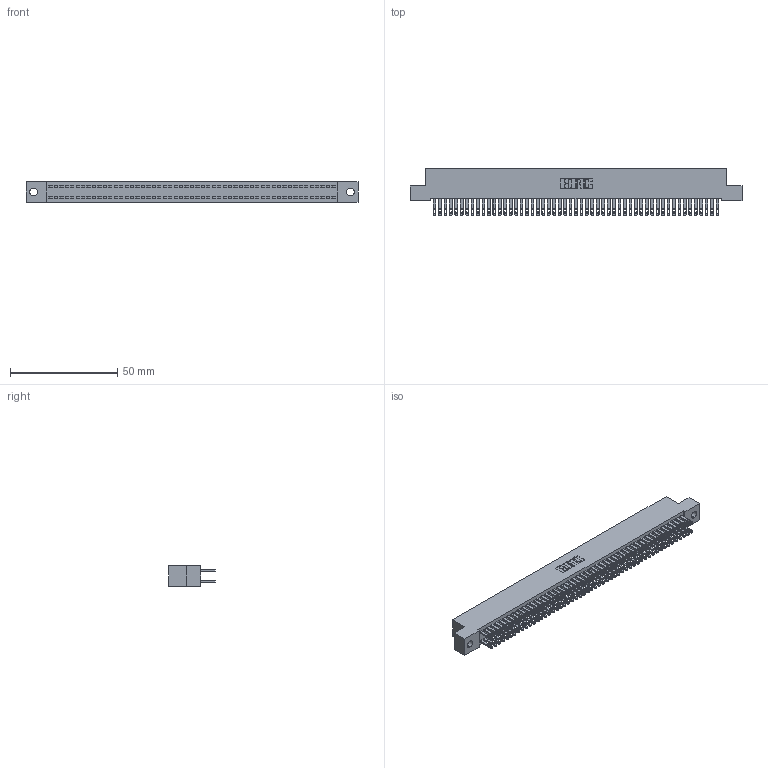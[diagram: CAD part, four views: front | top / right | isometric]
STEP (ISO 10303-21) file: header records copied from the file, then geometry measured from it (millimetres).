
FILE_DESCRIPTION (( 'STEP AP203' ), '1' );
FILE_NAME ('342-106-500-202.STEP', '2018-08-14T06:37:18', ( '' ), ( '' ), 'SwSTEP 2.0', 'SolidWorks 2016', '' );
FILE_SCHEMA (( 'CONFIG_CONTROL_DESIGN' ));
Length unit declared in the file: inch
Products named in the file (3): 345-292-001_345-293-100; 342-106-500-202; 342 Part_.128 Slot
Assembly tree (107 placements, depth 2):
  342-106-500-202
    342 Part_.128 Slot
    345-292-001_345-293-100  x106
Bounding box: 154.94 x 21.85 x 9.4 mm (x, y, z)
Volume: 14245.2 mm3; surface area: 24233 mm2
Topology: 107 solids, 107 shells, 5202 faces, 15893 edges, 10594 vertices
Faces by surface type: plane 3250, cylinder 1952
Entity records: 32607 total; most frequent: CARTESIAN_POINT 5390, ORIENTED_EDGE 5326, DIRECTION 4587, EDGE_CURVE 2663, LINE 2531, VECTOR 2531, VERTEX_POINT 1774, AXIS2_PLACEMENT_3D 1028
